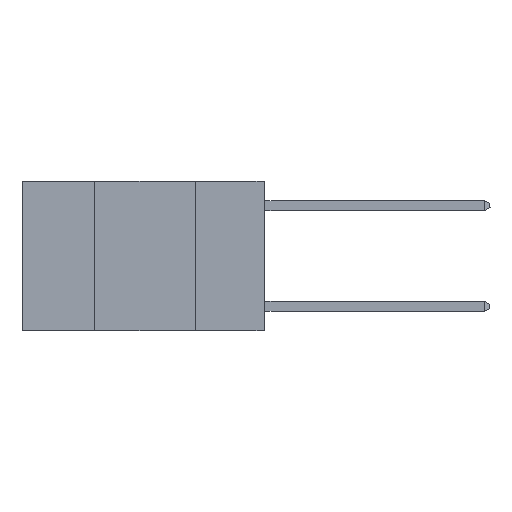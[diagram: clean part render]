
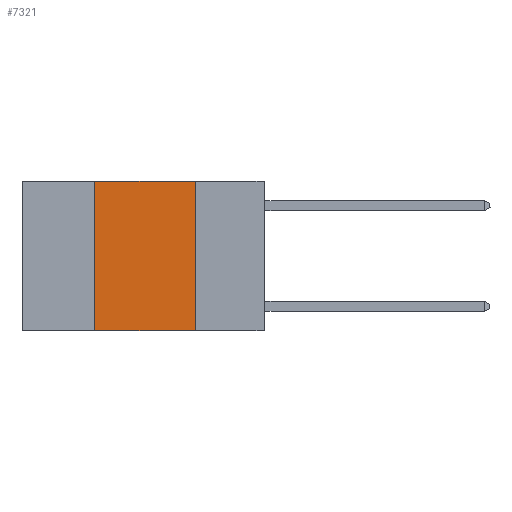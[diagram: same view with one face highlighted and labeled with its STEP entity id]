
A CAD part, left-side view. The second image highlights one B-rep face of the part: STEP entity #7321.
In plain terms, the highlighted planar face has unit normal (-1, 0, 0).
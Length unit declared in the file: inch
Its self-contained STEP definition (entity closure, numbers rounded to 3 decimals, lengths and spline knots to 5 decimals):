
#10 = DIRECTION ( 'NONE',  ( 0., -1., 0. ) ) ;
#999 = LINE ( 'NONE', #20371, #15346 ) ;
#1457 = DIRECTION ( 'NONE',  ( 1., 0., 0. ) ) ;
#1571 = AXIS2_PLACEMENT_3D ( 'NONE', #10831, #1457, #14548 ) ;
#3140 = ORIENTED_EDGE ( 'NONE', *, *, #21760, .F. ) ;
#3808 = CARTESIAN_POINT ( 'NONE',  ( 0., 0.42, 0. ) ) ;
#4327 = ORIENTED_EDGE ( 'NONE', *, *, #18037, .F. ) ;
#5522 = DIRECTION ( 'NONE',  ( 0., -1., 0. ) ) ;
#7321 = ADVANCED_FACE ( 'NONE', ( #14890 ), #12689, .F. ) ;
#7357 = DIRECTION ( 'NONE',  ( 0., 0., 1. ) ) ;
#7975 = EDGE_LOOP ( 'NONE', ( #3140, #23472, #4327, #9884 ) ) ;
#8566 = VECTOR ( 'NONE', #7357, 39.37008 ) ;
#9086 = CARTESIAN_POINT ( 'NONE',  ( 0., 0.17, -0.37 ) ) ;
#9341 = VERTEX_POINT ( 'NONE', #3808 ) ;
#9601 = LINE ( 'NONE', #23979, #13953 ) ;
#9884 = ORIENTED_EDGE ( 'NONE', *, *, #14331, .T. ) ;
#10831 = CARTESIAN_POINT ( 'NONE',  ( 0., 0.6, 0. ) ) ;
#11160 = DIRECTION ( 'NONE',  ( 0., 0., -1. ) ) ;
#12478 = EDGE_CURVE ( 'NONE', #9341, #18758, #9601, .T. ) ;
#12689 = PLANE ( 'NONE',  #1571 ) ;
#13953 = VECTOR ( 'NONE', #5522, 39.37008 ) ;
#14088 = LINE ( 'NONE', #18432, #8566 ) ;
#14331 = EDGE_CURVE ( 'NONE', #18175, #20985, #23420, .T. ) ;
#14548 = DIRECTION ( 'NONE',  ( 0., 0., -1. ) ) ;
#14890 = FACE_OUTER_BOUND ( 'NONE', #7975, .T. ) ;
#15124 = CARTESIAN_POINT ( 'NONE',  ( 0., 0.42, -0.37 ) ) ;
#15346 = VECTOR ( 'NONE', #11160, 39.37008 ) ;
#18037 = EDGE_CURVE ( 'NONE', #18175, #9341, #14088, .T. ) ;
#18175 = VERTEX_POINT ( 'NONE', #15124 ) ;
#18432 = CARTESIAN_POINT ( 'NONE',  ( 0., 0.42, 0. ) ) ;
#18564 = CARTESIAN_POINT ( 'NONE',  ( 0., 0.17, 0. ) ) ;
#18595 = CARTESIAN_POINT ( 'NONE',  ( 0., 0.6, -0.37 ) ) ;
#18758 = VERTEX_POINT ( 'NONE', #18564 ) ;
#20371 = CARTESIAN_POINT ( 'NONE',  ( 0., 0.17, 0. ) ) ;
#20985 = VERTEX_POINT ( 'NONE', #9086 ) ;
#21760 = EDGE_CURVE ( 'NONE', #18758, #20985, #999, .T. ) ;
#22850 = VECTOR ( 'NONE', #10, 39.37008 ) ;
#23420 = LINE ( 'NONE', #18595, #22850 ) ;
#23472 = ORIENTED_EDGE ( 'NONE', *, *, #12478, .F. ) ;
#23979 = CARTESIAN_POINT ( 'NONE',  ( 0., 0.6, 0. ) ) ;
